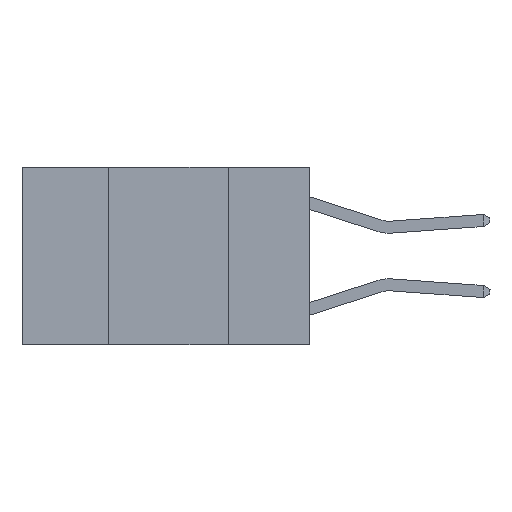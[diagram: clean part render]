
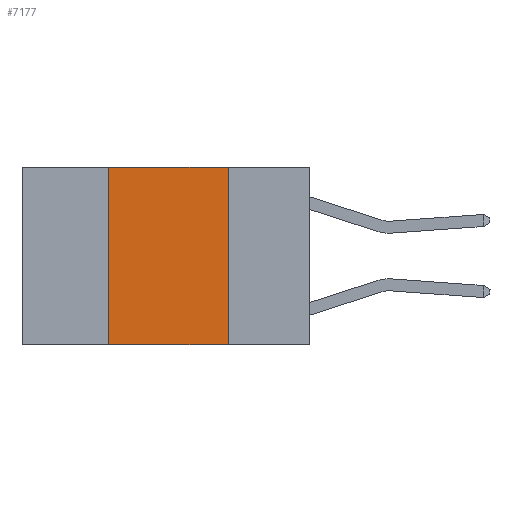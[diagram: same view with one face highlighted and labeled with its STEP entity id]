
A CAD part, left-side view. The second image highlights one B-rep face of the part: STEP entity #7177.
In plain terms, the highlighted planar face has unit normal (-1, 0, 0).
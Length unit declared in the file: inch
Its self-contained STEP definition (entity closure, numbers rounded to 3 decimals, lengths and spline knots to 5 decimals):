
#445 = CARTESIAN_POINT ( 'NONE',  ( 0., 0.17, 0. ) ) ;
#508 = EDGE_LOOP ( 'NONE', ( #7071, #9244, #6683, #1881 ) ) ;
#534 = CARTESIAN_POINT ( 'NONE',  ( 0., 0.6, -0.37 ) ) ;
#810 = EDGE_CURVE ( 'NONE', #6192, #1290, #7838, .T. ) ;
#1034 = VECTOR ( 'NONE', #8382, 39.37008 ) ;
#1290 = VERTEX_POINT ( 'NONE', #2046 ) ;
#1393 = CARTESIAN_POINT ( 'NONE',  ( 0., 0.6, 0. ) ) ;
#1881 = ORIENTED_EDGE ( 'NONE', *, *, #12155, .T. ) ;
#1900 = VERTEX_POINT ( 'NONE', #6974 ) ;
#2046 = CARTESIAN_POINT ( 'NONE',  ( 0., 0.17, -0.37 ) ) ;
#2480 = PLANE ( 'NONE',  #11444 ) ;
#2583 = VERTEX_POINT ( 'NONE', #7064 ) ;
#2952 = LINE ( 'NONE', #1393, #7231 ) ;
#3319 = EDGE_CURVE ( 'NONE', #2583, #1900, #11624, .T. ) ;
#3487 = DIRECTION ( 'NONE',  ( 1., 0., 0. ) ) ;
#3685 = LINE ( 'NONE', #534, #1034 ) ;
#5337 = DIRECTION ( 'NONE',  ( 0., -1., 0. ) ) ;
#6076 = DIRECTION ( 'NONE',  ( 0., 0., -1. ) ) ;
#6192 = VERTEX_POINT ( 'NONE', #11519 ) ;
#6498 = VECTOR ( 'NONE', #9130, 39.37008 ) ;
#6683 = ORIENTED_EDGE ( 'NONE', *, *, #3319, .F. ) ;
#6974 = CARTESIAN_POINT ( 'NONE',  ( 0., 0.42, 0. ) ) ;
#7064 = CARTESIAN_POINT ( 'NONE',  ( 0., 0.42, -0.37 ) ) ;
#7071 = ORIENTED_EDGE ( 'NONE', *, *, #810, .F. ) ;
#7177 = ADVANCED_FACE ( 'NONE', ( #11970 ), #2480, .F. ) ;
#7231 = VECTOR ( 'NONE', #5337, 39.37008 ) ;
#7838 = LINE ( 'NONE', #445, #10094 ) ;
#8329 = CARTESIAN_POINT ( 'NONE',  ( 0., 0.6, 0. ) ) ;
#8382 = DIRECTION ( 'NONE',  ( 0., -1., 0. ) ) ;
#9130 = DIRECTION ( 'NONE',  ( 0., 0., 1. ) ) ;
#9244 = ORIENTED_EDGE ( 'NONE', *, *, #10756, .F. ) ;
#9551 = CARTESIAN_POINT ( 'NONE',  ( 0., 0.42, 0. ) ) ;
#10094 = VECTOR ( 'NONE', #6076, 39.37008 ) ;
#10268 = DIRECTION ( 'NONE',  ( 0., 0., -1. ) ) ;
#10756 = EDGE_CURVE ( 'NONE', #1900, #6192, #2952, .T. ) ;
#11444 = AXIS2_PLACEMENT_3D ( 'NONE', #8329, #3487, #10268 ) ;
#11519 = CARTESIAN_POINT ( 'NONE',  ( 0., 0.17, 0. ) ) ;
#11624 = LINE ( 'NONE', #9551, #6498 ) ;
#11970 = FACE_OUTER_BOUND ( 'NONE', #508, .T. ) ;
#12155 = EDGE_CURVE ( 'NONE', #2583, #1290, #3685, .T. ) ;
